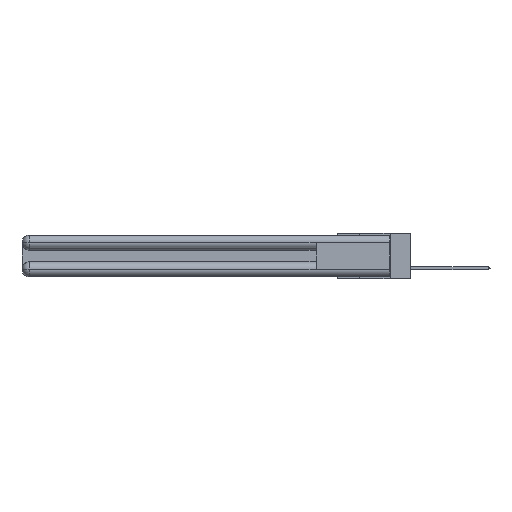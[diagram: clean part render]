
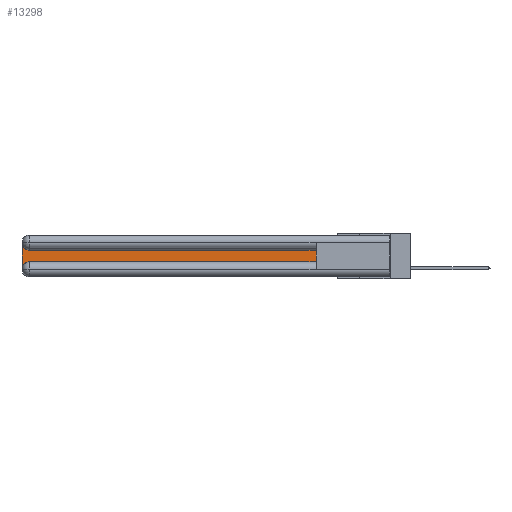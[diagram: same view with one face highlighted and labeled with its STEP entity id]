
A CAD part, left-side view. The second image highlights one B-rep face of the part: STEP entity #13298.
In plain terms, the highlighted planar face has unit normal (-1, 0, 0).
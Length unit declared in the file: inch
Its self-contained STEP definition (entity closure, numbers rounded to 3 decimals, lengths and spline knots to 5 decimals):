
#521 = ORIENTED_EDGE ( 'NONE', *, *, #7794, .T. ) ;
#708 = ORIENTED_EDGE ( 'NONE', *, *, #10255, .T. ) ;
#886 = VECTOR ( 'NONE', #6536, 39.37008 ) ;
#1358 = AXIS2_PLACEMENT_3D ( 'NONE', #13122, #25339, #28253 ) ;
#2896 = DIRECTION ( 'NONE',  ( 0., 0., -1. ) ) ;
#4039 = EDGE_CURVE ( 'NONE', #23578, #29680, #10213, .T. ) ;
#4502 = CARTESIAN_POINT ( 'NONE',  ( 0.075, 3., -0.2775 ) ) ;
#4895 = VECTOR ( 'NONE', #18986, 39.37008 ) ;
#5336 = PLANE ( 'NONE',  #27752 ) ;
#6219 = LINE ( 'NONE', #20435, #15707 ) ;
#6536 = DIRECTION ( 'NONE',  ( 0., 1., 0. ) ) ;
#7151 = LINE ( 'NONE', #13614, #24515 ) ;
#7794 = EDGE_CURVE ( 'NONE', #21028, #23578, #7151, .T. ) ;
#8777 = DIRECTION ( 'NONE',  ( 0., 0., -1. ) ) ;
#9498 = CIRCLE ( 'NONE', #1358, 0.06 ) ;
#10213 = CIRCLE ( 'NONE', #32005, 0.06 ) ;
#10255 = EDGE_CURVE ( 'NONE', #19956, #21028, #9498, .T. ) ;
#10472 = ORIENTED_EDGE ( 'NONE', *, *, #19153, .T. ) ;
#10553 = CARTESIAN_POINT ( 'NONE',  ( 0.075, 0.6, -0.2175 ) ) ;
#11009 = EDGE_CURVE ( 'NONE', #29680, #11037, #6219, .T. ) ;
#11037 = VERTEX_POINT ( 'NONE', #10553 ) ;
#11133 = EDGE_LOOP ( 'NONE', ( #10472, #708, #521, #24247, #29624, #24656 ) ) ;
#11709 = CARTESIAN_POINT ( 'NONE',  ( 0.075, 0.6, -0.1225 ) ) ;
#12475 = LINE ( 'NONE', #21402, #4895 ) ;
#12534 = EDGE_CURVE ( 'NONE', #11037, #24508, #12475, .T. ) ;
#13122 = CARTESIAN_POINT ( 'NONE',  ( 0.075, 2.94, -0.0625 ) ) ;
#13298 = ADVANCED_FACE ( 'NONE', ( #32145 ), #5336, .F. ) ;
#13614 = CARTESIAN_POINT ( 'NONE',  ( 0.075, 3., -0.2175 ) ) ;
#14056 = CARTESIAN_POINT ( 'NONE',  ( 0.075, 3., -0.0625 ) ) ;
#15633 = CARTESIAN_POINT ( 'NONE',  ( 0.075, 3., -0.1225 ) ) ;
#15707 = VECTOR ( 'NONE', #20553, 39.37008 ) ;
#18986 = DIRECTION ( 'NONE',  ( 0., 0., 1. ) ) ;
#19153 = EDGE_CURVE ( 'NONE', #24508, #19956, #20642, .T. ) ;
#19956 = VERTEX_POINT ( 'NONE', #28848 ) ;
#20435 = CARTESIAN_POINT ( 'NONE',  ( 0.075, 0.6, -0.2175 ) ) ;
#20553 = DIRECTION ( 'NONE',  ( 0., -1., 0. ) ) ;
#20642 = LINE ( 'NONE', #21632, #886 ) ;
#21028 = VERTEX_POINT ( 'NONE', #14056 ) ;
#21402 = CARTESIAN_POINT ( 'NONE',  ( 0.075, 0.6, -0.2175 ) ) ;
#21632 = CARTESIAN_POINT ( 'NONE',  ( 0.075, 0.6, -0.1225 ) ) ;
#21731 = CARTESIAN_POINT ( 'NONE',  ( 0.075, 2.94, -0.2175 ) ) ;
#21967 = DIRECTION ( 'NONE',  ( 1., 0., 0. ) ) ;
#22894 = DIRECTION ( 'NONE',  ( 1., 0., 0. ) ) ;
#23578 = VERTEX_POINT ( 'NONE', #4502 ) ;
#24247 = ORIENTED_EDGE ( 'NONE', *, *, #4039, .T. ) ;
#24508 = VERTEX_POINT ( 'NONE', #11709 ) ;
#24515 = VECTOR ( 'NONE', #8777, 39.37008 ) ;
#24656 = ORIENTED_EDGE ( 'NONE', *, *, #12534, .T. ) ;
#25339 = DIRECTION ( 'NONE',  ( 1., 0., 0. ) ) ;
#27752 = AXIS2_PLACEMENT_3D ( 'NONE', #15633, #22894, #2896 ) ;
#28253 = DIRECTION ( 'NONE',  ( 0., 0., -1. ) ) ;
#28848 = CARTESIAN_POINT ( 'NONE',  ( 0.075, 2.94, -0.1225 ) ) ;
#29195 = CARTESIAN_POINT ( 'NONE',  ( 0.075, 2.94, -0.2775 ) ) ;
#29301 = DIRECTION ( 'NONE',  ( 0., 0., -1. ) ) ;
#29624 = ORIENTED_EDGE ( 'NONE', *, *, #11009, .T. ) ;
#29680 = VERTEX_POINT ( 'NONE', #21731 ) ;
#32005 = AXIS2_PLACEMENT_3D ( 'NONE', #29195, #21967, #29301 ) ;
#32145 = FACE_OUTER_BOUND ( 'NONE', #11133, .T. ) ;
